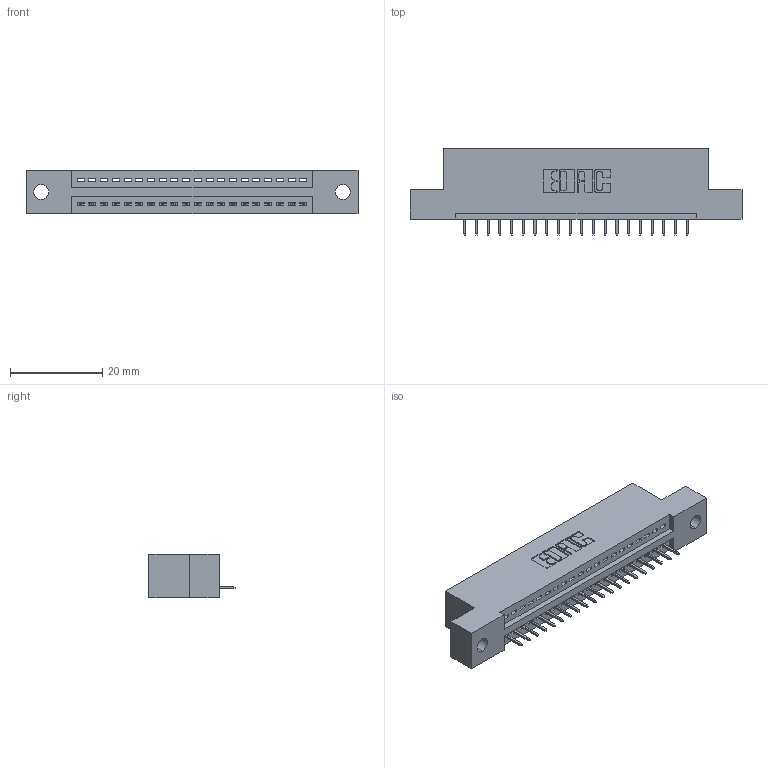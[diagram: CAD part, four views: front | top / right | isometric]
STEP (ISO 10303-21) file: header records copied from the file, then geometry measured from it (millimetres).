
FILE_DESCRIPTION (( 'STEP AP203' ), '1' );
FILE_NAME ('345-020-525-102.STEP', '2020-09-19T05:19:22', ( '' ), ( '' ), 'SwSTEP 2.0', 'SolidWorks 2020', '' );
FILE_SCHEMA (( 'CONFIG_CONTROL_DESIGN' ));
Length unit declared in the file: inch
Products named in the file (3): 345-292-001_345-293-125; 345 Part_Flush Mounting Lugs - 0.128 Dia; 345-020-525-102
Assembly tree (21 placements, depth 2):
  345-020-525-102
    345 Part_Flush Mounting Lugs - 0.128 Dia
    345-292-001_345-293-125  x20
Bounding box: 72.01 x 18.72 x 9.4 mm (x, y, z)
Volume: 6540.9 mm3; surface area: 7849.5 mm2
Topology: 21 solids, 21 shells, 1366 faces, 3941 edges, 2546 vertices
Faces by surface type: plane 1000, cylinder 366
Entity records: 18091 total; most frequent: CARTESIAN_POINT 3140, ORIENTED_EDGE 3094, DIRECTION 2775, EDGE_CURVE 1547, LINE 1339, VECTOR 1339, VERTEX_POINT 1026, AXIS2_PLACEMENT_3D 718
